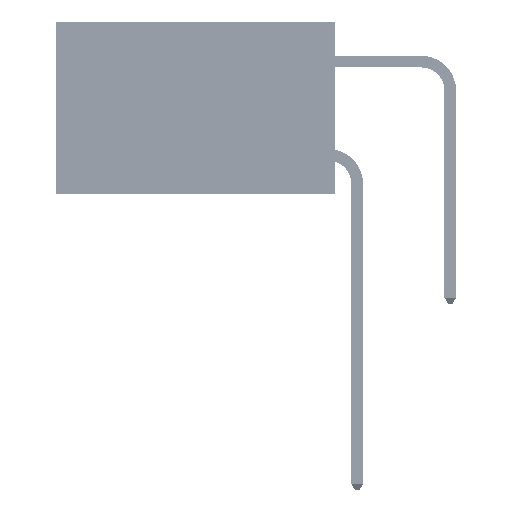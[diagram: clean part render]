
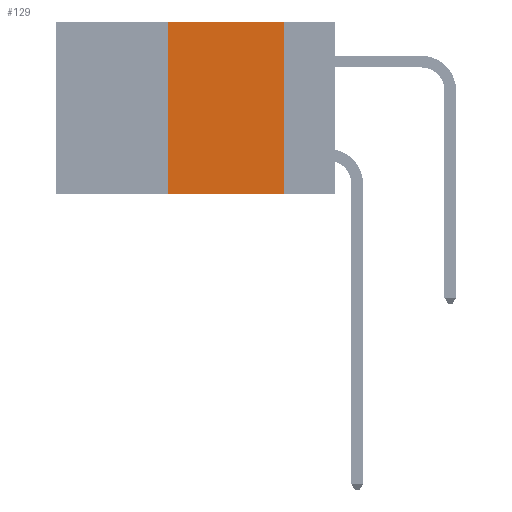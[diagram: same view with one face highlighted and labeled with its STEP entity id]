
A CAD part, left-side view. The second image highlights one B-rep face of the part: STEP entity #129.
In plain terms, the highlighted planar face has unit normal (-1, 0, 0).
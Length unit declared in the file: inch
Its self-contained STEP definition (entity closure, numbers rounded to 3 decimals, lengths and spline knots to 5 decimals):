
#129 = ADVANCED_FACE ( 'NONE', ( #8801 ), #44533, .F. ) ;
#2103 = CARTESIAN_POINT ( 'NONE',  ( 0., 0.36, -0.37 ) ) ;
#2532 = CARTESIAN_POINT ( 'NONE',  ( 0., 0.6, 0. ) ) ;
#3817 = EDGE_CURVE ( 'NONE', #47050, #20951, #12843, .T. ) ;
#5774 = ORIENTED_EDGE ( 'NONE', *, *, #3817, .T. ) ;
#5883 = LINE ( 'NONE', #12787, #32532 ) ;
#8801 = FACE_OUTER_BOUND ( 'NONE', #15460, .T. ) ;
#10078 = DIRECTION ( 'NONE',  ( 0., 0., -1. ) ) ;
#10416 = CARTESIAN_POINT ( 'NONE',  ( 0., 0.11, 0. ) ) ;
#12341 = VERTEX_POINT ( 'NONE', #17769 ) ;
#12787 = CARTESIAN_POINT ( 'NONE',  ( 0., 0.36, 0. ) ) ;
#12843 = LINE ( 'NONE', #16592, #37166 ) ;
#12897 = VECTOR ( 'NONE', #10078, 39.37008 ) ;
#14089 = LINE ( 'NONE', #10416, #12897 ) ;
#15460 = EDGE_LOOP ( 'NONE', ( #40965, #31543, #41153, #5774 ) ) ;
#15880 = LINE ( 'NONE', #2532, #32503 ) ;
#16592 = CARTESIAN_POINT ( 'NONE',  ( 0., 0.6, -0.37 ) ) ;
#16710 = EDGE_CURVE ( 'NONE', #47050, #12341, #5883, .T. ) ;
#17769 = CARTESIAN_POINT ( 'NONE',  ( 0., 0.36, 0. ) ) ;
#18008 = DIRECTION ( 'NONE',  ( 1., 0., 0. ) ) ;
#19767 = DIRECTION ( 'NONE',  ( 0., -1., 0. ) ) ;
#20951 = VERTEX_POINT ( 'NONE', #24348 ) ;
#21232 = CARTESIAN_POINT ( 'NONE',  ( 0., 0.11, 0. ) ) ;
#21820 = DIRECTION ( 'NONE',  ( 0., 0., -1. ) ) ;
#24348 = CARTESIAN_POINT ( 'NONE',  ( 0., 0.11, -0.37 ) ) ;
#25336 = CARTESIAN_POINT ( 'NONE',  ( 0., 0.6, 0. ) ) ;
#31543 = ORIENTED_EDGE ( 'NONE', *, *, #40942, .F. ) ;
#32503 = VECTOR ( 'NONE', #44251, 39.37008 ) ;
#32532 = VECTOR ( 'NONE', #35653, 39.37008 ) ;
#35653 = DIRECTION ( 'NONE',  ( 0., 0., 1. ) ) ;
#37166 = VECTOR ( 'NONE', #19767, 39.37008 ) ;
#38466 = VERTEX_POINT ( 'NONE', #21232 ) ;
#40942 = EDGE_CURVE ( 'NONE', #12341, #38466, #15880, .T. ) ;
#40965 = ORIENTED_EDGE ( 'NONE', *, *, #41676, .F. ) ;
#41153 = ORIENTED_EDGE ( 'NONE', *, *, #16710, .F. ) ;
#41676 = EDGE_CURVE ( 'NONE', #38466, #20951, #14089, .T. ) ;
#44251 = DIRECTION ( 'NONE',  ( 0., -1., 0. ) ) ;
#44533 = PLANE ( 'NONE',  #45145 ) ;
#45145 = AXIS2_PLACEMENT_3D ( 'NONE', #25336, #18008, #21820 ) ;
#47050 = VERTEX_POINT ( 'NONE', #2103 ) ;
